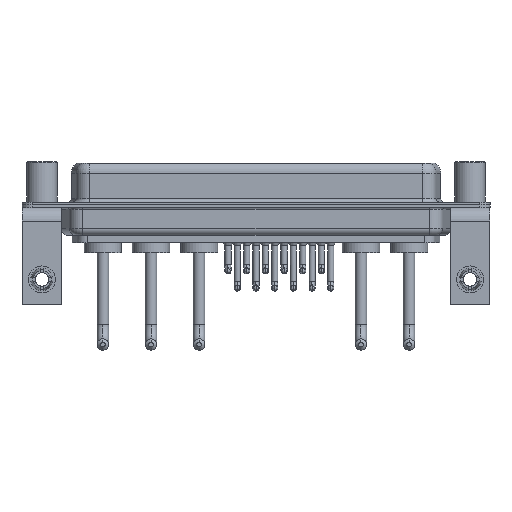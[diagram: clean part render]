
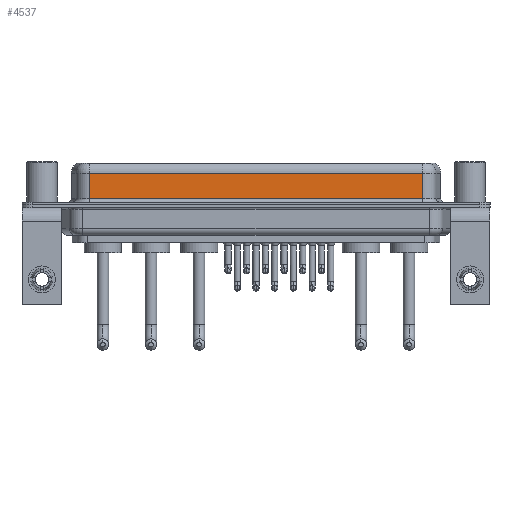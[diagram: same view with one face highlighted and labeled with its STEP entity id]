
A CAD part, front view. The second image highlights one B-rep face of the part: STEP entity #4537.
In plain terms, the highlighted planar face has unit normal (0, -1, 0).
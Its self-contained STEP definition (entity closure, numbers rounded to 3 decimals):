
#138 = DIRECTION ( 'NONE',  ( 0., 0., 1. ) ) ;
#256 = EDGE_CURVE ( 'NONE', #15622, #8070, #14215, .T. ) ;
#931 = VECTOR ( 'NONE', #19356, 1000. ) ;
#1938 = FACE_OUTER_BOUND ( 'NONE', #8753, .T. ) ;
#3849 = CARTESIAN_POINT ( 'NONE',  ( 7.038, -3.95, 4.65 ) ) ;
#3985 = PLANE ( 'NONE',  #7779 ) ;
#4364 = ORIENTED_EDGE ( 'NONE', *, *, #19821, .T. ) ;
#4537 = ADVANCED_FACE ( 'NONE', ( #1938 ), #3985, .F. ) ;
#5076 = CARTESIAN_POINT ( 'NONE',  ( 56.462, -3.95, 4.65 ) ) ;
#5734 = VECTOR ( 'NONE', #7231, 1000. ) ;
#6728 = DIRECTION ( 'NONE',  ( 0., 0., -1. ) ) ;
#7075 = CARTESIAN_POINT ( 'NONE',  ( 56.462, -3.95, 0.9 ) ) ;
#7231 = DIRECTION ( 'NONE',  ( -1., 0., 0. ) ) ;
#7779 = AXIS2_PLACEMENT_3D ( 'NONE', #13354, #9734, #138 ) ;
#8070 = VERTEX_POINT ( 'NONE', #3849 ) ;
#8753 = EDGE_LOOP ( 'NONE', ( #13740, #19346, #12881, #4364 ) ) ;
#9734 = DIRECTION ( 'NONE',  ( 0., 1., 0. ) ) ;
#9894 = VECTOR ( 'NONE', #23252, 1000. ) ;
#9924 = EDGE_CURVE ( 'NONE', #15622, #20344, #10324, .T. ) ;
#10324 = LINE ( 'NONE', #23435, #23262 ) ;
#12186 = CARTESIAN_POINT ( 'NONE',  ( 7.038, -3.95, 6.4 ) ) ;
#12881 = ORIENTED_EDGE ( 'NONE', *, *, #13733, .T. ) ;
#13354 = CARTESIAN_POINT ( 'NONE',  ( 56.462, -3.95, 6.4 ) ) ;
#13733 = EDGE_CURVE ( 'NONE', #8070, #16507, #15921, .T. ) ;
#13740 = ORIENTED_EDGE ( 'NONE', *, *, #9924, .F. ) ;
#14215 = LINE ( 'NONE', #5076, #5734 ) ;
#14290 = CARTESIAN_POINT ( 'NONE',  ( 56.462, -3.95, 0.9 ) ) ;
#15622 = VERTEX_POINT ( 'NONE', #21894 ) ;
#15921 = LINE ( 'NONE', #12186, #9894 ) ;
#16306 = CARTESIAN_POINT ( 'NONE',  ( 7.038, -3.95, 0.9 ) ) ;
#16507 = VERTEX_POINT ( 'NONE', #16306 ) ;
#19346 = ORIENTED_EDGE ( 'NONE', *, *, #256, .T. ) ;
#19356 = DIRECTION ( 'NONE',  ( 1., 0., 0. ) ) ;
#19821 = EDGE_CURVE ( 'NONE', #16507, #20344, #21513, .T. ) ;
#20344 = VERTEX_POINT ( 'NONE', #14290 ) ;
#21513 = LINE ( 'NONE', #7075, #931 ) ;
#21894 = CARTESIAN_POINT ( 'NONE',  ( 56.462, -3.95, 4.65 ) ) ;
#23252 = DIRECTION ( 'NONE',  ( 0., 0., -1. ) ) ;
#23262 = VECTOR ( 'NONE', #6728, 1000. ) ;
#23435 = CARTESIAN_POINT ( 'NONE',  ( 56.462, -3.95, 6.4 ) ) ;
